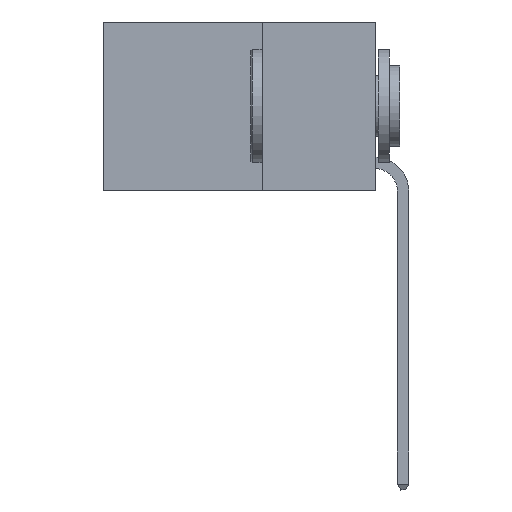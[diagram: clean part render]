
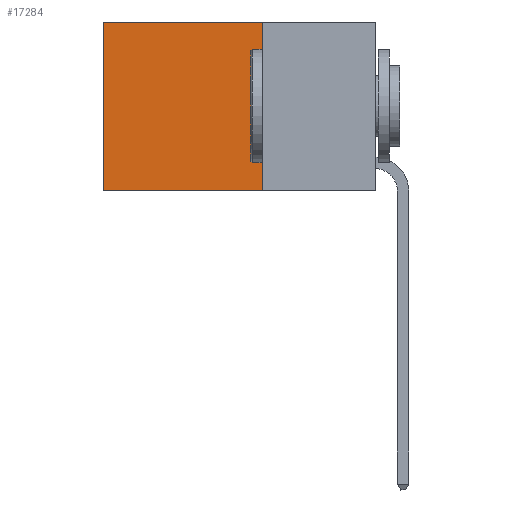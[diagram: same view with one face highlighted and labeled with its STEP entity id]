
A CAD part, left-side view. The second image highlights one B-rep face of the part: STEP entity #17284.
In plain terms, the highlighted planar face has unit normal (-1, 0, 0).
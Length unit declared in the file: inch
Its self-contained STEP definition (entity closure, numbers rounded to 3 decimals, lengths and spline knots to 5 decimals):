
#513 = VECTOR ( 'NONE', #13971, 39.37008 ) ;
#1449 = LINE ( 'NONE', #5647, #7134 ) ;
#1928 = DIRECTION ( 'NONE',  ( 0., 1., 0. ) ) ;
#3294 = VECTOR ( 'NONE', #11189, 39.37008 ) ;
#4598 = CARTESIAN_POINT ( 'NONE',  ( 0.2625, 0.25, 0. ) ) ;
#5647 = CARTESIAN_POINT ( 'NONE',  ( 0.2625, 0.25, 0. ) ) ;
#5739 = CARTESIAN_POINT ( 'NONE',  ( 0.2625, 0.25, -0.37 ) ) ;
#5806 = ORIENTED_EDGE ( 'NONE', *, *, #6821, .T. ) ;
#6821 = EDGE_CURVE ( 'NONE', #13454, #25996, #24056, .T. ) ;
#7043 = VECTOR ( 'NONE', #1928, 39.37008 ) ;
#7134 = VECTOR ( 'NONE', #16461, 39.37008 ) ;
#8512 = CARTESIAN_POINT ( 'NONE',  ( 0.2625, 0.25, 0. ) ) ;
#8784 = DIRECTION ( 'NONE',  ( 1., 0., 0. ) ) ;
#10834 = EDGE_CURVE ( 'NONE', #20619, #13454, #19734, .T. ) ;
#11189 = DIRECTION ( 'NONE',  ( 0., 1., 0. ) ) ;
#13454 = VERTEX_POINT ( 'NONE', #25988 ) ;
#13971 = DIRECTION ( 'NONE',  ( 0., 0., -1. ) ) ;
#14224 = AXIS2_PLACEMENT_3D ( 'NONE', #8512, #8784, #17077 ) ;
#14424 = CARTESIAN_POINT ( 'NONE',  ( 0.2625, 0.25, -0.37 ) ) ;
#15462 = CARTESIAN_POINT ( 'NONE',  ( 0.2625, 0.25, 0. ) ) ;
#15523 = PLANE ( 'NONE',  #14224 ) ;
#16461 = DIRECTION ( 'NONE',  ( 0., 0., -1. ) ) ;
#17077 = DIRECTION ( 'NONE',  ( 0., 0., -1. ) ) ;
#17284 = ADVANCED_FACE ( 'NONE', ( #19173 ), #15523, .F. ) ;
#17550 = ORIENTED_EDGE ( 'NONE', *, *, #25062, .F. ) ;
#18008 = ORIENTED_EDGE ( 'NONE', *, *, #10834, .T. ) ;
#18300 = VERTEX_POINT ( 'NONE', #5739 ) ;
#18681 = EDGE_LOOP ( 'NONE', ( #5806, #17550, #24712, #18008 ) ) ;
#19173 = FACE_OUTER_BOUND ( 'NONE', #18681, .T. ) ;
#19734 = LINE ( 'NONE', #4598, #3294 ) ;
#20619 = VERTEX_POINT ( 'NONE', #15462 ) ;
#22703 = LINE ( 'NONE', #14424, #7043 ) ;
#24056 = LINE ( 'NONE', #24183, #513 ) ;
#24183 = CARTESIAN_POINT ( 'NONE',  ( 0.2625, 0.6, 0. ) ) ;
#24712 = ORIENTED_EDGE ( 'NONE', *, *, #27110, .F. ) ;
#25062 = EDGE_CURVE ( 'NONE', #18300, #25996, #22703, .T. ) ;
#25557 = CARTESIAN_POINT ( 'NONE',  ( 0.2625, 0.6, -0.37 ) ) ;
#25988 = CARTESIAN_POINT ( 'NONE',  ( 0.2625, 0.6, 0. ) ) ;
#25996 = VERTEX_POINT ( 'NONE', #25557 ) ;
#27110 = EDGE_CURVE ( 'NONE', #20619, #18300, #1449, .T. ) ;
